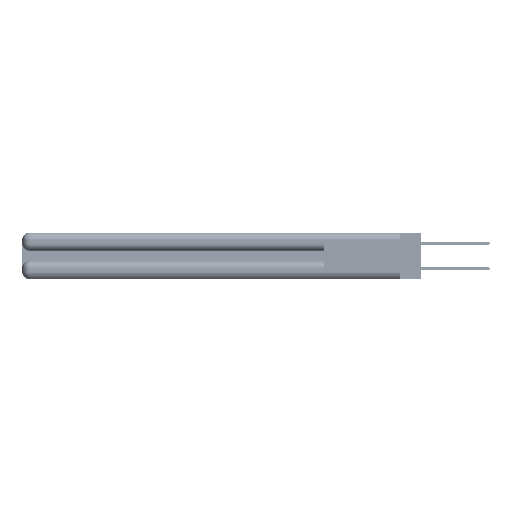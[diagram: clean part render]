
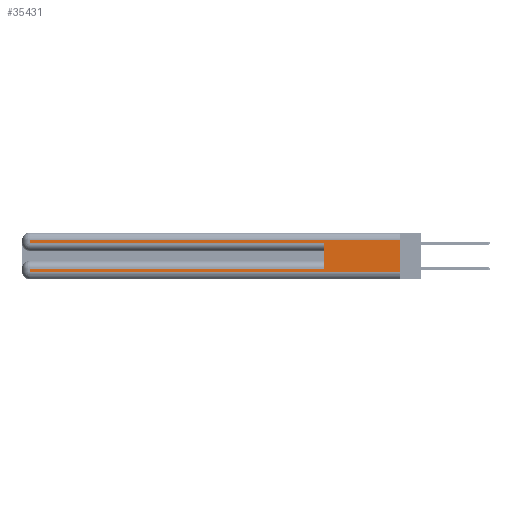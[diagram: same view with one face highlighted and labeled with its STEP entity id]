
A CAD part, left-side view. The second image highlights one B-rep face of the part: STEP entity #35431.
In plain terms, the highlighted planar face has unit normal (-1, 0, 0).
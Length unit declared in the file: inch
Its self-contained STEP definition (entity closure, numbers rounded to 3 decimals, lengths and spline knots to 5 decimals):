
#1474 = LINE ( 'NONE', #15793, #11741 ) ;
#1759 = VECTOR ( 'NONE', #41940, 39.37008 ) ;
#1879 = CARTESIAN_POINT ( 'NONE',  ( 0., 2.94, 0.06 ) ) ;
#2565 = EDGE_LOOP ( 'NONE', ( #18271, #21059, #49044, #32073, #55181, #23893, #38812, #16934 ) ) ;
#3562 = EDGE_CURVE ( 'NONE', #37486, #26214, #13381, .T. ) ;
#4047 = AXIS2_PLACEMENT_3D ( 'NONE', #7848, #38429, #12241 ) ;
#4490 = VECTOR ( 'NONE', #53280, 39.37008 ) ;
#4869 = VECTOR ( 'NONE', #28388, 39.37008 ) ;
#5081 = EDGE_CURVE ( 'NONE', #47328, #54467, #7733, .T. ) ;
#5615 = VERTEX_POINT ( 'NONE', #33546 ) ;
#6972 = CARTESIAN_POINT ( 'NONE',  ( 0., 0., 0.285 ) ) ;
#7733 = LINE ( 'NONE', #42943, #10483 ) ;
#7848 = CARTESIAN_POINT ( 'NONE',  ( 0., 0., 0.37 ) ) ;
#8616 = VECTOR ( 'NONE', #25561, 39.37008 ) ;
#9861 = FACE_OUTER_BOUND ( 'NONE', #2565, .T. ) ;
#10483 = VECTOR ( 'NONE', #16762, 39.37008 ) ;
#11585 = CARTESIAN_POINT ( 'NONE',  ( 0., 0., 0.37 ) ) ;
#11741 = VECTOR ( 'NONE', #20206, 39.37008 ) ;
#12241 = DIRECTION ( 'NONE',  ( 0., 0., -1. ) ) ;
#12491 = CARTESIAN_POINT ( 'NONE',  ( 0., 0., 0.31 ) ) ;
#13097 = DIRECTION ( 'NONE',  ( 0., 1., 0. ) ) ;
#13381 = LINE ( 'NONE', #6972, #1759 ) ;
#15793 = CARTESIAN_POINT ( 'NONE',  ( 0., 0., 0.31 ) ) ;
#16139 = LINE ( 'NONE', #40178, #4490 ) ;
#16762 = DIRECTION ( 'NONE',  ( 0., -1., 0. ) ) ;
#16934 = ORIENTED_EDGE ( 'NONE', *, *, #5081, .T. ) ;
#18271 = ORIENTED_EDGE ( 'NONE', *, *, #23367, .F. ) ;
#18577 = EDGE_CURVE ( 'NONE', #34795, #47475, #1474, .T. ) ;
#18825 = CARTESIAN_POINT ( 'NONE',  ( 0., 0., 0.06 ) ) ;
#19979 = LINE ( 'NONE', #39280, #43200 ) ;
#20206 = DIRECTION ( 'NONE',  ( 0., 1., 0. ) ) ;
#21059 = ORIENTED_EDGE ( 'NONE', *, *, #18577, .T. ) ;
#21966 = EDGE_CURVE ( 'NONE', #5615, #47328, #16139, .T. ) ;
#23367 = EDGE_CURVE ( 'NONE', #34795, #54467, #36226, .T. ) ;
#23893 = ORIENTED_EDGE ( 'NONE', *, *, #43498, .T. ) ;
#24004 = CARTESIAN_POINT ( 'NONE',  ( 0., 2.94, 0.37 ) ) ;
#25293 = PLANE ( 'NONE',  #4047 ) ;
#25561 = DIRECTION ( 'NONE',  ( 0., 0., 1. ) ) ;
#26214 = VERTEX_POINT ( 'NONE', #29901 ) ;
#28388 = DIRECTION ( 'NONE',  ( 0., 0., -1. ) ) ;
#29901 = CARTESIAN_POINT ( 'NONE',  ( 0., 0.6, 0.285 ) ) ;
#31923 = LINE ( 'NONE', #38508, #8616 ) ;
#32073 = ORIENTED_EDGE ( 'NONE', *, *, #3562, .T. ) ;
#33546 = CARTESIAN_POINT ( 'NONE',  ( 0., 2.94, 0.085 ) ) ;
#34795 = VERTEX_POINT ( 'NONE', #12491 ) ;
#35431 = ADVANCED_FACE ( 'NONE', ( #9861 ), #25293, .F. ) ;
#36226 = LINE ( 'NONE', #11585, #37564 ) ;
#37486 = VERTEX_POINT ( 'NONE', #45167 ) ;
#37564 = VECTOR ( 'NONE', #42146, 39.37008 ) ;
#38429 = DIRECTION ( 'NONE',  ( 1., 0., 0. ) ) ;
#38508 = CARTESIAN_POINT ( 'NONE',  ( 0., 0.6, 0.145 ) ) ;
#38812 = ORIENTED_EDGE ( 'NONE', *, *, #21966, .T. ) ;
#39280 = CARTESIAN_POINT ( 'NONE',  ( 0., 0., 0.085 ) ) ;
#39747 = LINE ( 'NONE', #24004, #4869 ) ;
#40178 = CARTESIAN_POINT ( 'NONE',  ( 0., 2.94, 0.37 ) ) ;
#41778 = VERTEX_POINT ( 'NONE', #41938 ) ;
#41938 = CARTESIAN_POINT ( 'NONE',  ( 0., 0.6, 0.085 ) ) ;
#41940 = DIRECTION ( 'NONE',  ( 0., -1., 0. ) ) ;
#42146 = DIRECTION ( 'NONE',  ( 0., 0., -1. ) ) ;
#42943 = CARTESIAN_POINT ( 'NONE',  ( 0., 0., 0.06 ) ) ;
#43200 = VECTOR ( 'NONE', #13097, 39.37008 ) ;
#43498 = EDGE_CURVE ( 'NONE', #41778, #5615, #19979, .T. ) ;
#43824 = EDGE_CURVE ( 'NONE', #47475, #37486, #39747, .T. ) ;
#45167 = CARTESIAN_POINT ( 'NONE',  ( 0., 2.94, 0.285 ) ) ;
#47328 = VERTEX_POINT ( 'NONE', #1879 ) ;
#47475 = VERTEX_POINT ( 'NONE', #50735 ) ;
#49044 = ORIENTED_EDGE ( 'NONE', *, *, #43824, .T. ) ;
#50735 = CARTESIAN_POINT ( 'NONE',  ( 0., 2.94, 0.31 ) ) ;
#53280 = DIRECTION ( 'NONE',  ( 0., 0., -1. ) ) ;
#54467 = VERTEX_POINT ( 'NONE', #18825 ) ;
#55181 = ORIENTED_EDGE ( 'NONE', *, *, #56200, .F. ) ;
#56200 = EDGE_CURVE ( 'NONE', #41778, #26214, #31923, .T. ) ;
